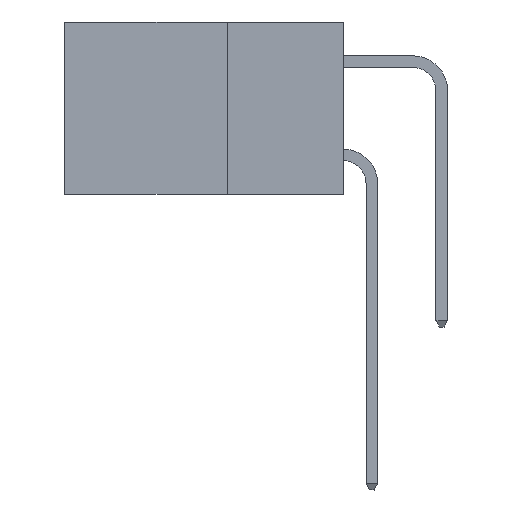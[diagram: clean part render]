
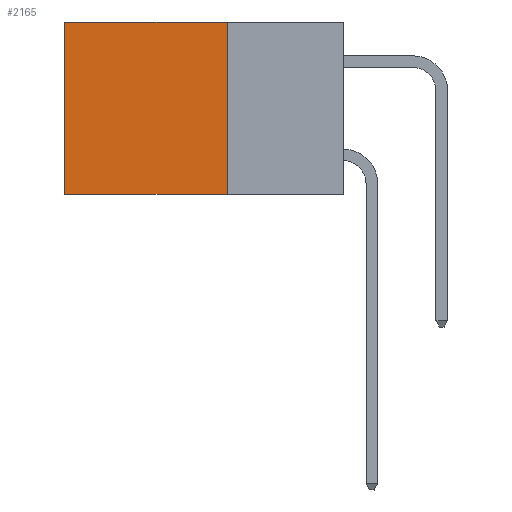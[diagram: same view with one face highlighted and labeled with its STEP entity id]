
A CAD part, left-side view. The second image highlights one B-rep face of the part: STEP entity #2165.
In plain terms, the highlighted planar face has unit normal (-1, 0, 0).
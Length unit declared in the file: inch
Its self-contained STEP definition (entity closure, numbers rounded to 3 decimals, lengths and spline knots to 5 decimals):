
#171 = EDGE_LOOP ( 'NONE', ( #2262, #9602, #9512, #2131 ) ) ;
#191 = LINE ( 'NONE', #7568, #12342 ) ;
#352 = PLANE ( 'NONE',  #7801 ) ;
#393 = LINE ( 'NONE', #6355, #5456 ) ;
#516 = CARTESIAN_POINT ( 'NONE',  ( 0.298, 0.6, -0.37 ) ) ;
#577 = DIRECTION ( 'NONE',  ( 1., 0., 0. ) ) ;
#1685 = CARTESIAN_POINT ( 'NONE',  ( 0.298, 0.25, 0. ) ) ;
#1687 = CARTESIAN_POINT ( 'NONE',  ( 0.298, 0.25, 0. ) ) ;
#1971 = CARTESIAN_POINT ( 'NONE',  ( 0.298, 0.6, 0. ) ) ;
#1991 = EDGE_CURVE ( 'NONE', #3745, #11697, #10300, .T. ) ;
#2131 = ORIENTED_EDGE ( 'NONE', *, *, #3011, .T. ) ;
#2165 = ADVANCED_FACE ( 'NONE', ( #7973 ), #352, .F. ) ;
#2262 = ORIENTED_EDGE ( 'NONE', *, *, #7255, .T. ) ;
#2549 = DIRECTION ( 'NONE',  ( 0., 1., 0. ) ) ;
#3011 = EDGE_CURVE ( 'NONE', #3745, #7644, #4622, .T. ) ;
#3293 = EDGE_CURVE ( 'NONE', #11697, #7905, #191, .T. ) ;
#3745 = VERTEX_POINT ( 'NONE', #1685 ) ;
#4622 = LINE ( 'NONE', #9721, #9546 ) ;
#5456 = VECTOR ( 'NONE', #7361, 39.37008 ) ;
#6355 = CARTESIAN_POINT ( 'NONE',  ( 0.298, 0.6, 0. ) ) ;
#6945 = CARTESIAN_POINT ( 'NONE',  ( 0.298, 0.25, -0.37 ) ) ;
#7230 = CARTESIAN_POINT ( 'NONE',  ( 0.298, 0.25, 0. ) ) ;
#7255 = EDGE_CURVE ( 'NONE', #7644, #7905, #393, .T. ) ;
#7361 = DIRECTION ( 'NONE',  ( 0., 0., -1. ) ) ;
#7517 = VECTOR ( 'NONE', #7831, 39.37008 ) ;
#7568 = CARTESIAN_POINT ( 'NONE',  ( 0.298, 0.25, -0.37 ) ) ;
#7605 = DIRECTION ( 'NONE',  ( 0., 0., -1. ) ) ;
#7644 = VERTEX_POINT ( 'NONE', #1971 ) ;
#7801 = AXIS2_PLACEMENT_3D ( 'NONE', #1687, #577, #7605 ) ;
#7831 = DIRECTION ( 'NONE',  ( 0., 0., -1. ) ) ;
#7905 = VERTEX_POINT ( 'NONE', #516 ) ;
#7973 = FACE_OUTER_BOUND ( 'NONE', #171, .T. ) ;
#9512 = ORIENTED_EDGE ( 'NONE', *, *, #1991, .F. ) ;
#9546 = VECTOR ( 'NONE', #2549, 39.37008 ) ;
#9602 = ORIENTED_EDGE ( 'NONE', *, *, #3293, .F. ) ;
#9721 = CARTESIAN_POINT ( 'NONE',  ( 0.298, 0.25, 0. ) ) ;
#9800 = DIRECTION ( 'NONE',  ( 0., 1., 0. ) ) ;
#10300 = LINE ( 'NONE', #7230, #7517 ) ;
#11697 = VERTEX_POINT ( 'NONE', #6945 ) ;
#12342 = VECTOR ( 'NONE', #9800, 39.37008 ) ;
